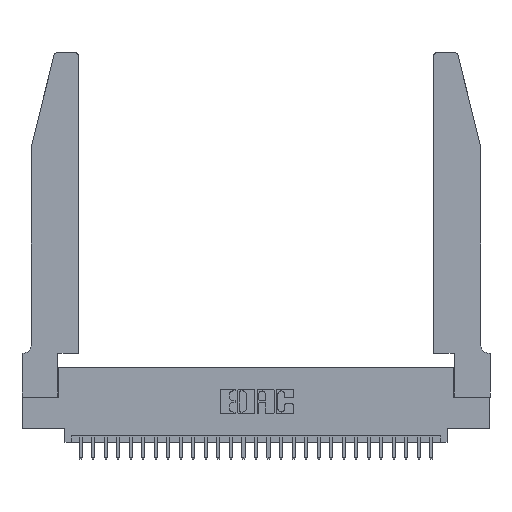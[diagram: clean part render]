
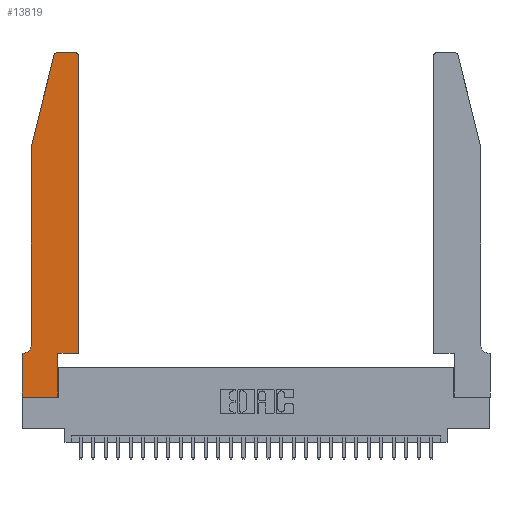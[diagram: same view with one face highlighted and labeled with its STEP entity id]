
A CAD part, top view. The second image highlights one B-rep face of the part: STEP entity #13819.
In plain terms, the highlighted planar face has unit normal (0, 0, 1).
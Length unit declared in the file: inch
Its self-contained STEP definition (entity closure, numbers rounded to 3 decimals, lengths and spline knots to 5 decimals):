
#576 = VERTEX_POINT ( 'NONE', #16097 ) ;
#1432 = EDGE_CURVE ( 'NONE', #6937, #17057, #10383, .T. ) ;
#1916 = DIRECTION ( 'NONE',  ( -0.239, -0.971, 0. ) ) ;
#1966 = VERTEX_POINT ( 'NONE', #19602 ) ;
#2203 = CARTESIAN_POINT ( 'NONE',  ( 0.4505, 0.35, 0.37 ) ) ;
#2470 = DIRECTION ( 'NONE',  ( 0., 0., 1. ) ) ;
#2638 = CARTESIAN_POINT ( 'NONE',  ( 0.2605, 2.75, 0.37 ) ) ;
#2909 = VERTEX_POINT ( 'NONE', #21338 ) ;
#2952 = VECTOR ( 'NONE', #15852, 39.37008 ) ;
#3045 = VERTEX_POINT ( 'NONE', #19450 ) ;
#3248 = LINE ( 'NONE', #12240, #14659 ) ;
#3350 = DIRECTION ( 'NONE',  ( 1., 0., 0. ) ) ;
#3404 = EDGE_LOOP ( 'NONE', ( #12851, #14276, #14968, #20981, #23083, #6515, #7246, #20646, #22749, #12198, #24149, #18876 ) ) ;
#3980 = VECTOR ( 'NONE', #19422, 39.37008 ) ;
#4575 = AXIS2_PLACEMENT_3D ( 'NONE', #16141, #2470, #18395 ) ;
#5862 = CIRCLE ( 'NONE', #4575, 0.03 ) ;
#6062 = DIRECTION ( 'NONE',  ( 0., 1., 0. ) ) ;
#6161 = CARTESIAN_POINT ( 'NONE',  ( 0.4505, 0.35, 0.37 ) ) ;
#6371 = VERTEX_POINT ( 'NONE', #2203 ) ;
#6515 = ORIENTED_EDGE ( 'NONE', *, *, #11000, .T. ) ;
#6626 = LINE ( 'NONE', #21622, #11620 ) ;
#6937 = VERTEX_POINT ( 'NONE', #7008 ) ;
#7008 = CARTESIAN_POINT ( 'NONE',  ( 0.4505, 2.72, 0.37 ) ) ;
#7059 = VECTOR ( 'NONE', #8870, 39.37008 ) ;
#7246 = ORIENTED_EDGE ( 'NONE', *, *, #22086, .T. ) ;
#7478 = CARTESIAN_POINT ( 'NONE',  ( 0., 0., 0.37 ) ) ;
#7493 = EDGE_CURVE ( 'NONE', #1966, #13303, #5862, .T. ) ;
#8870 = DIRECTION ( 'NONE',  ( -1., 0., 0. ) ) ;
#8974 = EDGE_CURVE ( 'NONE', #576, #2909, #3248, .T. ) ;
#10369 = EDGE_CURVE ( 'NONE', #3045, #11908, #20576, .T. ) ;
#10383 = CIRCLE ( 'NONE', #21779, 0.03 ) ;
#10518 = LINE ( 'NONE', #20470, #27727 ) ;
#10863 = DIRECTION ( 'NONE',  ( 0., 0., -1. ) ) ;
#11000 = EDGE_CURVE ( 'NONE', #11908, #21210, #12359, .T. ) ;
#11620 = VECTOR ( 'NONE', #26089, 39.37008 ) ;
#11893 = FACE_OUTER_BOUND ( 'NONE', #3404, .T. ) ;
#11908 = VERTEX_POINT ( 'NONE', #21141 ) ;
#12198 = ORIENTED_EDGE ( 'NONE', *, *, #12982, .T. ) ;
#12240 = CARTESIAN_POINT ( 'NONE',  ( 0.2865, 0.35, 0.37 ) ) ;
#12359 = LINE ( 'NONE', #22359, #7059 ) ;
#12740 = VERTEX_POINT ( 'NONE', #21778 ) ;
#12851 = ORIENTED_EDGE ( 'NONE', *, *, #29270, .T. ) ;
#12982 = EDGE_CURVE ( 'NONE', #2909, #6371, #26996, .T. ) ;
#13071 = VECTOR ( 'NONE', #20949, 39.37008 ) ;
#13104 = DIRECTION ( 'NONE',  ( 0., 0., 1. ) ) ;
#13303 = VERTEX_POINT ( 'NONE', #21453 ) ;
#13589 = CARTESIAN_POINT ( 'NONE',  ( 0.4505, 0.35, 0.37 ) ) ;
#13613 = AXIS2_PLACEMENT_3D ( 'NONE', #15269, #13104, #28798 ) ;
#13819 = ADVANCED_FACE ( 'NONE', ( #11893 ), #22075, .T. ) ;
#14276 = ORIENTED_EDGE ( 'NONE', *, *, #7493, .T. ) ;
#14489 = DIRECTION ( 'NONE',  ( 0., 1., 0. ) ) ;
#14659 = VECTOR ( 'NONE', #14489, 39.37008 ) ;
#14968 = ORIENTED_EDGE ( 'NONE', *, *, #16449, .T. ) ;
#15269 = CARTESIAN_POINT ( 'NONE',  ( 0., 0.35, 0.37 ) ) ;
#15852 = DIRECTION ( 'NONE',  ( 1., 0., 0. ) ) ;
#16097 = CARTESIAN_POINT ( 'NONE',  ( 0.2865, 0., 0.37 ) ) ;
#16141 = CARTESIAN_POINT ( 'NONE',  ( 0.284, 2.72, 0.37 ) ) ;
#16449 = EDGE_CURVE ( 'NONE', #13303, #12740, #27144, .T. ) ;
#16654 = CARTESIAN_POINT ( 'NONE',  ( 0., 0.35, 0.37 ) ) ;
#16768 = AXIS2_PLACEMENT_3D ( 'NONE', #24343, #10863, #26552 ) ;
#17057 = VERTEX_POINT ( 'NONE', #28841 ) ;
#17544 = EDGE_CURVE ( 'NONE', #12740, #3045, #27271, .T. ) ;
#17548 = CARTESIAN_POINT ( 'NONE',  ( 0.4205, 2.72, 0.37 ) ) ;
#17902 = CARTESIAN_POINT ( 'NONE',  ( 0.0755, 2., 0.37 ) ) ;
#18395 = DIRECTION ( 'NONE',  ( 1., 0., 0. ) ) ;
#18518 = VERTEX_POINT ( 'NONE', #7478 ) ;
#18876 = ORIENTED_EDGE ( 'NONE', *, *, #1432, .T. ) ;
#19075 = LINE ( 'NONE', #2638, #13071 ) ;
#19422 = DIRECTION ( 'NONE',  ( 0., -1., 0. ) ) ;
#19450 = CARTESIAN_POINT ( 'NONE',  ( 0.0755, 0.42, 0.37 ) ) ;
#19602 = CARTESIAN_POINT ( 'NONE',  ( 0.284, 2.75, 0.37 ) ) ;
#20470 = CARTESIAN_POINT ( 'NONE',  ( 0., 0., 0.37 ) ) ;
#20576 = CIRCLE ( 'NONE', #16768, 0.07 ) ;
#20646 = ORIENTED_EDGE ( 'NONE', *, *, #21661, .T. ) ;
#20949 = DIRECTION ( 'NONE',  ( -1., 0., 0. ) ) ;
#20969 = DIRECTION ( 'NONE',  ( 0., 0., 1. ) ) ;
#20981 = ORIENTED_EDGE ( 'NONE', *, *, #17544, .T. ) ;
#21141 = CARTESIAN_POINT ( 'NONE',  ( 0.0055, 0.35, 0.37 ) ) ;
#21210 = VERTEX_POINT ( 'NONE', #16654 ) ;
#21338 = CARTESIAN_POINT ( 'NONE',  ( 0.2865, 0.35, 0.37 ) ) ;
#21453 = CARTESIAN_POINT ( 'NONE',  ( 0.25487, 2.72718, 0.37 ) ) ;
#21622 = CARTESIAN_POINT ( 'NONE',  ( 0., 0., 0.37 ) ) ;
#21661 = EDGE_CURVE ( 'NONE', #18518, #576, #10518, .T. ) ;
#21778 = CARTESIAN_POINT ( 'NONE',  ( 0.0755, 2., 0.37 ) ) ;
#21779 = AXIS2_PLACEMENT_3D ( 'NONE', #17548, #20969, #3350 ) ;
#22075 = PLANE ( 'NONE',  #13613 ) ;
#22086 = EDGE_CURVE ( 'NONE', #21210, #18518, #6626, .T. ) ;
#22359 = CARTESIAN_POINT ( 'NONE',  ( 0.0755, 0.35, 0.37 ) ) ;
#22644 = VECTOR ( 'NONE', #1916, 39.37008 ) ;
#22729 = DIRECTION ( 'NONE',  ( 1., 0., 0. ) ) ;
#22749 = ORIENTED_EDGE ( 'NONE', *, *, #8974, .T. ) ;
#23083 = ORIENTED_EDGE ( 'NONE', *, *, #10369, .T. ) ;
#23675 = VECTOR ( 'NONE', #6062, 39.37008 ) ;
#23946 = CARTESIAN_POINT ( 'NONE',  ( 0.0755, 2., 0.37 ) ) ;
#24149 = ORIENTED_EDGE ( 'NONE', *, *, #28878, .T. ) ;
#24343 = CARTESIAN_POINT ( 'NONE',  ( 0.0055, 0.42, 0.37 ) ) ;
#26089 = DIRECTION ( 'NONE',  ( 0., -1., 0. ) ) ;
#26552 = DIRECTION ( 'NONE',  ( -1., 0., 0. ) ) ;
#26996 = LINE ( 'NONE', #13589, #2952 ) ;
#27144 = LINE ( 'NONE', #17902, #22644 ) ;
#27271 = LINE ( 'NONE', #23946, #3980 ) ;
#27727 = VECTOR ( 'NONE', #22729, 39.37008 ) ;
#28798 = DIRECTION ( 'NONE',  ( 1., 0., 0. ) ) ;
#28841 = CARTESIAN_POINT ( 'NONE',  ( 0.4205, 2.75, 0.37 ) ) ;
#28878 = EDGE_CURVE ( 'NONE', #6371, #6937, #28902, .T. ) ;
#28902 = LINE ( 'NONE', #6161, #23675 ) ;
#29270 = EDGE_CURVE ( 'NONE', #17057, #1966, #19075, .T. ) ;
